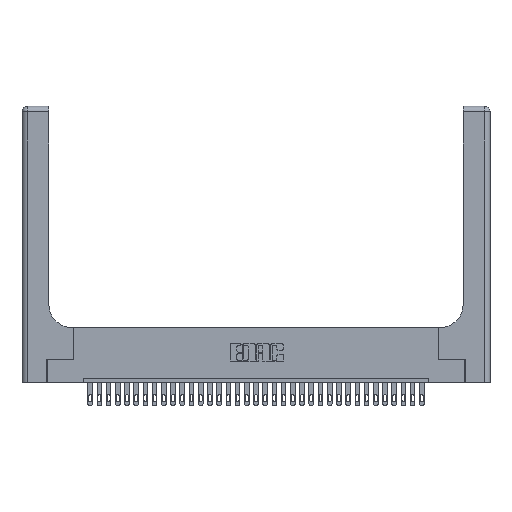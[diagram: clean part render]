
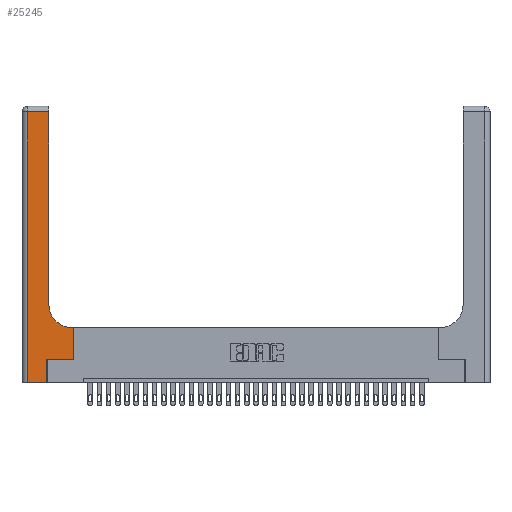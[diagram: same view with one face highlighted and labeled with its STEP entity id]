
A CAD part, top view. The second image highlights one B-rep face of the part: STEP entity #25245.
In plain terms, the highlighted planar face has unit normal (0, 0, 1).
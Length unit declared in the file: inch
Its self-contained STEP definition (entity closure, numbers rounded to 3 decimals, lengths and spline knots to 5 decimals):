
#116 = EDGE_LOOP ( 'NONE', ( #9957, #22895, #3592, #22364, #7573, #21065, #2400, #11193, #8538 ) ) ;
#287 = AXIS2_PLACEMENT_3D ( 'NONE', #22371, #32698, #1511 ) ;
#561 = LINE ( 'NONE', #1259, #1409 ) ;
#906 = VERTEX_POINT ( 'NONE', #28371 ) ;
#1219 = VECTOR ( 'NONE', #29208, 39.37008 ) ;
#1259 = CARTESIAN_POINT ( 'NONE',  ( 0.269, 0., 0.37 ) ) ;
#1323 = EDGE_CURVE ( 'NONE', #2393, #18570, #7196, .T. ) ;
#1409 = VECTOR ( 'NONE', #13806, 39.37008 ) ;
#1511 = DIRECTION ( 'NONE',  ( -1., 0., 0. ) ) ;
#1535 = VERTEX_POINT ( 'NONE', #31161 ) ;
#1663 = CIRCLE ( 'NONE', #4432, 0.25 ) ;
#2190 = EDGE_CURVE ( 'NONE', #18570, #19293, #561, .T. ) ;
#2313 = VECTOR ( 'NONE', #25039, 39.37008 ) ;
#2393 = VERTEX_POINT ( 'NONE', #12402 ) ;
#2400 = ORIENTED_EDGE ( 'NONE', *, *, #2562, .T. ) ;
#2562 = EDGE_CURVE ( 'NONE', #18073, #20586, #15947, .T. ) ;
#2906 = CARTESIAN_POINT ( 'NONE',  ( 0.269, 0.25, 0.37 ) ) ;
#3592 = ORIENTED_EDGE ( 'NONE', *, *, #32244, .T. ) ;
#3787 = CARTESIAN_POINT ( 'NONE',  ( 0., 0., 0.37 ) ) ;
#4288 = DIRECTION ( 'NONE',  ( 0., 1., 0. ) ) ;
#4432 = AXIS2_PLACEMENT_3D ( 'NONE', #25347, #22858, #7317 ) ;
#5246 = CARTESIAN_POINT ( 'NONE',  ( 0.5585, 0.25, 0.37 ) ) ;
#5250 = CARTESIAN_POINT ( 'NONE',  ( 0.2915, 3., 0.37 ) ) ;
#5502 = VERTEX_POINT ( 'NONE', #13217 ) ;
#7064 = PLANE ( 'NONE',  #287 ) ;
#7196 = LINE ( 'NONE', #3787, #2313 ) ;
#7317 = DIRECTION ( 'NONE',  ( 1., 0., 0. ) ) ;
#7573 = ORIENTED_EDGE ( 'NONE', *, *, #2190, .T. ) ;
#8063 = LINE ( 'NONE', #11234, #1219 ) ;
#8538 = ORIENTED_EDGE ( 'NONE', *, *, #24745, .T. ) ;
#9424 = LINE ( 'NONE', #23382, #30979 ) ;
#9957 = ORIENTED_EDGE ( 'NONE', *, *, #20357, .T. ) ;
#11193 = ORIENTED_EDGE ( 'NONE', *, *, #17152, .T. ) ;
#11234 = CARTESIAN_POINT ( 'NONE',  ( 0.06, 3., 0.37 ) ) ;
#12402 = CARTESIAN_POINT ( 'NONE',  ( 0.06, 0., 0.37 ) ) ;
#12547 = CARTESIAN_POINT ( 'NONE',  ( 0.2915, 2.94, 0.37 ) ) ;
#13217 = CARTESIAN_POINT ( 'NONE',  ( 0.06, 2.94, 0.37 ) ) ;
#13311 = LINE ( 'NONE', #5250, #33265 ) ;
#13806 = DIRECTION ( 'NONE',  ( 0., 1., 0. ) ) ;
#15947 = LINE ( 'NONE', #27205, #21220 ) ;
#16829 = VECTOR ( 'NONE', #23855, 39.37008 ) ;
#17152 = EDGE_CURVE ( 'NONE', #20586, #906, #26960, .T. ) ;
#17221 = CARTESIAN_POINT ( 'NONE',  ( 0.269, 0., 0.37 ) ) ;
#18073 = VERTEX_POINT ( 'NONE', #5246 ) ;
#18383 = DIRECTION ( 'NONE',  ( 1., 0., 0. ) ) ;
#18570 = VERTEX_POINT ( 'NONE', #17221 ) ;
#18812 = CARTESIAN_POINT ( 'NONE',  ( 0.5585, 0.6, 0.37 ) ) ;
#19070 = VERTEX_POINT ( 'NONE', #12547 ) ;
#19293 = VERTEX_POINT ( 'NONE', #2906 ) ;
#20357 = EDGE_CURVE ( 'NONE', #1535, #19070, #13311, .T. ) ;
#20586 = VERTEX_POINT ( 'NONE', #18812 ) ;
#21065 = ORIENTED_EDGE ( 'NONE', *, *, #23469, .T. ) ;
#21220 = VECTOR ( 'NONE', #4288, 39.37008 ) ;
#22364 = ORIENTED_EDGE ( 'NONE', *, *, #1323, .T. ) ;
#22371 = CARTESIAN_POINT ( 'NONE',  ( 0., 3., 0.37 ) ) ;
#22858 = DIRECTION ( 'NONE',  ( 0., 0., -1. ) ) ;
#22895 = ORIENTED_EDGE ( 'NONE', *, *, #28638, .T. ) ;
#23382 = CARTESIAN_POINT ( 'NONE',  ( 0.269, 0.25, 0.37 ) ) ;
#23469 = EDGE_CURVE ( 'NONE', #19293, #18073, #9424, .T. ) ;
#23855 = DIRECTION ( 'NONE',  ( -1., 0., 0. ) ) ;
#24745 = EDGE_CURVE ( 'NONE', #906, #1535, #1663, .T. ) ;
#25039 = DIRECTION ( 'NONE',  ( 1., 0., 0. ) ) ;
#25245 = ADVANCED_FACE ( 'NONE', ( #32103 ), #7064, .F. ) ;
#25347 = CARTESIAN_POINT ( 'NONE',  ( 0.5415, 0.85, 0.37 ) ) ;
#25771 = CARTESIAN_POINT ( 'NONE',  ( 0., 2.94, 0.37 ) ) ;
#26473 = CARTESIAN_POINT ( 'NONE',  ( 0.2915, 0.6, 0.37 ) ) ;
#26960 = LINE ( 'NONE', #26473, #16829 ) ;
#27205 = CARTESIAN_POINT ( 'NONE',  ( 0.5585, 0.25, 0.37 ) ) ;
#28371 = CARTESIAN_POINT ( 'NONE',  ( 0.5415, 0.6, 0.37 ) ) ;
#28611 = VECTOR ( 'NONE', #30913, 39.37008 ) ;
#28638 = EDGE_CURVE ( 'NONE', #19070, #5502, #32715, .T. ) ;
#29208 = DIRECTION ( 'NONE',  ( 0., -1., 0. ) ) ;
#30913 = DIRECTION ( 'NONE',  ( -1., 0., 0. ) ) ;
#30979 = VECTOR ( 'NONE', #18383, 39.37008 ) ;
#31161 = CARTESIAN_POINT ( 'NONE',  ( 0.2915, 0.85, 0.37 ) ) ;
#32103 = FACE_OUTER_BOUND ( 'NONE', #116, .T. ) ;
#32244 = EDGE_CURVE ( 'NONE', #5502, #2393, #8063, .T. ) ;
#32698 = DIRECTION ( 'NONE',  ( 0., 0., -1. ) ) ;
#32715 = LINE ( 'NONE', #25771, #28611 ) ;
#33265 = VECTOR ( 'NONE', #33282, 39.37008 ) ;
#33282 = DIRECTION ( 'NONE',  ( 0., 1., 0. ) ) ;
